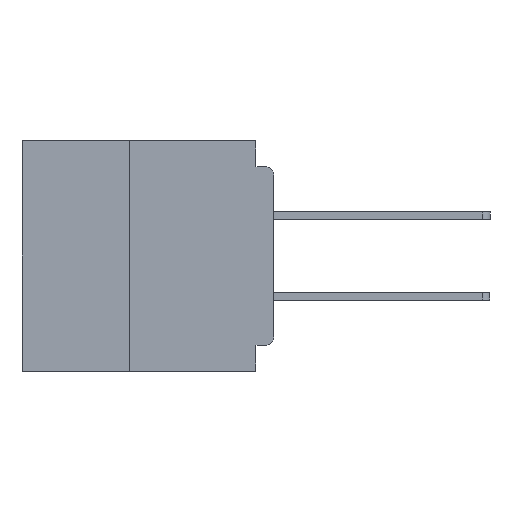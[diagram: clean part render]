
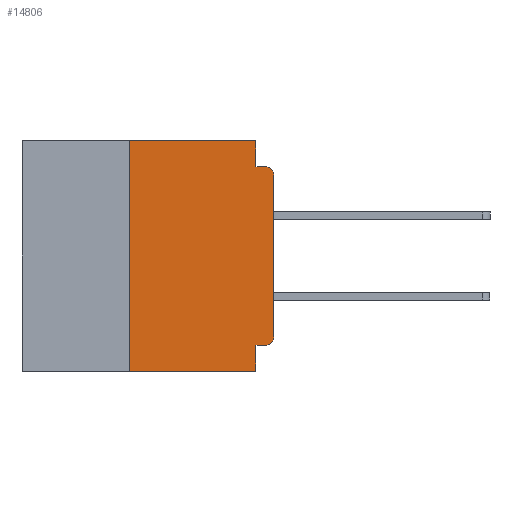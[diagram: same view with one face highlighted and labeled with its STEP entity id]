
A CAD part, left-side view. The second image highlights one B-rep face of the part: STEP entity #14806.
In plain terms, the highlighted planar face has unit normal (-1, 0, 0).
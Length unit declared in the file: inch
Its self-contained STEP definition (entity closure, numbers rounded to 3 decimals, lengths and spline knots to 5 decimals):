
#686 = EDGE_CURVE ( 'NONE', #10013, #43815, #5616, .T. ) ;
#1831 = CARTESIAN_POINT ( 'NONE',  ( 0., 0., -0.045 ) ) ;
#1938 = CARTESIAN_POINT ( 'NONE',  ( 0., 0., 0. ) ) ;
#2043 = CARTESIAN_POINT ( 'NONE',  ( 0., 0., -0.06 ) ) ;
#2425 = AXIS2_PLACEMENT_3D ( 'NONE', #49778, #26937, #3738 ) ;
#2740 = DIRECTION ( 'NONE',  ( 0., 0., -1. ) ) ;
#3738 = DIRECTION ( 'NONE',  ( 0., 0., -1. ) ) ;
#3967 = CARTESIAN_POINT ( 'NONE',  ( 0., 0., -0.34 ) ) ;
#5616 = CIRCLE ( 'NONE', #16342, 0.015 ) ;
#5784 = DIRECTION ( 'NONE',  ( 0., -1., 0. ) ) ;
#6579 = CARTESIAN_POINT ( 'NONE',  ( 0., 0., -0.355 ) ) ;
#7752 = LINE ( 'NONE', #1938, #47393 ) ;
#8097 = VECTOR ( 'NONE', #33523, 39.37008 ) ;
#8373 = VERTEX_POINT ( 'NONE', #30780 ) ;
#9880 = CARTESIAN_POINT ( 'NONE',  ( 0., 0.031, -0.045 ) ) ;
#10013 = VERTEX_POINT ( 'NONE', #2043 ) ;
#10057 = LINE ( 'NONE', #42242, #19170 ) ;
#10811 = ORIENTED_EDGE ( 'NONE', *, *, #44323, .T. ) ;
#12141 = CARTESIAN_POINT ( 'NONE',  ( 0., 0.437, 0. ) ) ;
#13792 = FACE_OUTER_BOUND ( 'NONE', #49432, .T. ) ;
#14806 = ADVANCED_FACE ( 'NONE', ( #13792 ), #19219, .F. ) ;
#14893 = DIRECTION ( 'NONE',  ( -1., 0., 0. ) ) ;
#15413 = CARTESIAN_POINT ( 'NONE',  ( 0., 0.25, -0.4 ) ) ;
#16158 = VECTOR ( 'NONE', #2740, 39.37008 ) ;
#16321 = ORIENTED_EDGE ( 'NONE', *, *, #686, .T. ) ;
#16342 = AXIS2_PLACEMENT_3D ( 'NONE', #29107, #26663, #26175 ) ;
#17948 = VERTEX_POINT ( 'NONE', #45543 ) ;
#18680 = ORIENTED_EDGE ( 'NONE', *, *, #34330, .F. ) ;
#18772 = VERTEX_POINT ( 'NONE', #35258 ) ;
#19170 = VECTOR ( 'NONE', #27046, 39.37008 ) ;
#19219 = PLANE ( 'NONE',  #2425 ) ;
#19724 = ORIENTED_EDGE ( 'NONE', *, *, #41225, .F. ) ;
#19936 = VERTEX_POINT ( 'NONE', #41317 ) ;
#19973 = DIRECTION ( 'NONE',  ( 0., -1., 0. ) ) ;
#20131 = ORIENTED_EDGE ( 'NONE', *, *, #49812, .T. ) ;
#20732 = EDGE_CURVE ( 'NONE', #23808, #8373, #10057, .T. ) ;
#23808 = VERTEX_POINT ( 'NONE', #15413 ) ;
#25969 = CARTESIAN_POINT ( 'NONE',  ( 0., 0.031, -0.4 ) ) ;
#26175 = DIRECTION ( 'NONE',  ( 0., 0., -1. ) ) ;
#26350 = LINE ( 'NONE', #12141, #45434 ) ;
#26421 = LINE ( 'NONE', #25969, #16158 ) ;
#26663 = DIRECTION ( 'NONE',  ( -1., 0., 0. ) ) ;
#26937 = DIRECTION ( 'NONE',  ( 1., 0., 0. ) ) ;
#26954 = CARTESIAN_POINT ( 'NONE',  ( 0., 0.437, -0.4 ) ) ;
#27046 = DIRECTION ( 'NONE',  ( 0., 0., 1. ) ) ;
#28871 = DIRECTION ( 'NONE',  ( 0., 0., 1. ) ) ;
#29107 = CARTESIAN_POINT ( 'NONE',  ( 0., 0.015, -0.06 ) ) ;
#30780 = CARTESIAN_POINT ( 'NONE',  ( 0., 0.25, 0. ) ) ;
#31041 = LINE ( 'NONE', #40302, #38800 ) ;
#31936 = EDGE_CURVE ( 'NONE', #18772, #17948, #26421, .T. ) ;
#32206 = CIRCLE ( 'NONE', #43655, 0.015 ) ;
#33523 = DIRECTION ( 'NONE',  ( 0., 1., 0. ) ) ;
#34330 = EDGE_CURVE ( 'NONE', #35104, #18772, #38782, .T. ) ;
#35104 = VERTEX_POINT ( 'NONE', #45949 ) ;
#35258 = CARTESIAN_POINT ( 'NONE',  ( 0., 0.031, -0.355 ) ) ;
#35356 = ORIENTED_EDGE ( 'NONE', *, *, #31936, .F. ) ;
#36614 = DIRECTION ( 'NONE',  ( 0., 0., -1. ) ) ;
#36709 = VECTOR ( 'NONE', #5784, 39.37008 ) ;
#37802 = ORIENTED_EDGE ( 'NONE', *, *, #20732, .F. ) ;
#37872 = CARTESIAN_POINT ( 'NONE',  ( 0., 0.015, -0.34 ) ) ;
#38090 = VECTOR ( 'NONE', #42320, 39.37008 ) ;
#38782 = LINE ( 'NONE', #6579, #8097 ) ;
#38800 = VECTOR ( 'NONE', #36614, 39.37008 ) ;
#39169 = ORIENTED_EDGE ( 'NONE', *, *, #40433, .F. ) ;
#39730 = ORIENTED_EDGE ( 'NONE', *, *, #43666, .F. ) ;
#40302 = CARTESIAN_POINT ( 'NONE',  ( 0., 0.031, 0. ) ) ;
#40433 = EDGE_CURVE ( 'NONE', #8373, #19936, #26350, .T. ) ;
#40759 = ORIENTED_EDGE ( 'NONE', *, *, #49049, .T. ) ;
#41225 = EDGE_CURVE ( 'NONE', #19936, #48234, #31041, .T. ) ;
#41263 = CARTESIAN_POINT ( 'NONE',  ( 0., 0.015, -0.045 ) ) ;
#41317 = CARTESIAN_POINT ( 'NONE',  ( 0., 0.031, 0. ) ) ;
#41728 = DIRECTION ( 'NONE',  ( 0., 0., -1. ) ) ;
#42242 = CARTESIAN_POINT ( 'NONE',  ( 0., 0.25, -0.4 ) ) ;
#42320 = DIRECTION ( 'NONE',  ( 0., -1., 0. ) ) ;
#42733 = VERTEX_POINT ( 'NONE', #3967 ) ;
#43655 = AXIS2_PLACEMENT_3D ( 'NONE', #37872, #14893, #41728 ) ;
#43666 = EDGE_CURVE ( 'NONE', #48234, #43815, #48052, .T. ) ;
#43815 = VERTEX_POINT ( 'NONE', #41263 ) ;
#44323 = EDGE_CURVE ( 'NONE', #42733, #10013, #7752, .T. ) ;
#45434 = VECTOR ( 'NONE', #19973, 39.37008 ) ;
#45543 = CARTESIAN_POINT ( 'NONE',  ( 0., 0.031, -0.4 ) ) ;
#45949 = CARTESIAN_POINT ( 'NONE',  ( 0., 0.015, -0.355 ) ) ;
#47393 = VECTOR ( 'NONE', #28871, 39.37008 ) ;
#48052 = LINE ( 'NONE', #1831, #36709 ) ;
#48214 = LINE ( 'NONE', #26954, #38090 ) ;
#48234 = VERTEX_POINT ( 'NONE', #9880 ) ;
#49049 = EDGE_CURVE ( 'NONE', #35104, #42733, #32206, .T. ) ;
#49432 = EDGE_LOOP ( 'NONE', ( #10811, #16321, #39730, #19724, #39169, #37802, #20131, #35356, #18680, #40759 ) ) ;
#49778 = CARTESIAN_POINT ( 'NONE',  ( 0., 0.437, 0. ) ) ;
#49812 = EDGE_CURVE ( 'NONE', #23808, #17948, #48214, .T. ) ;
